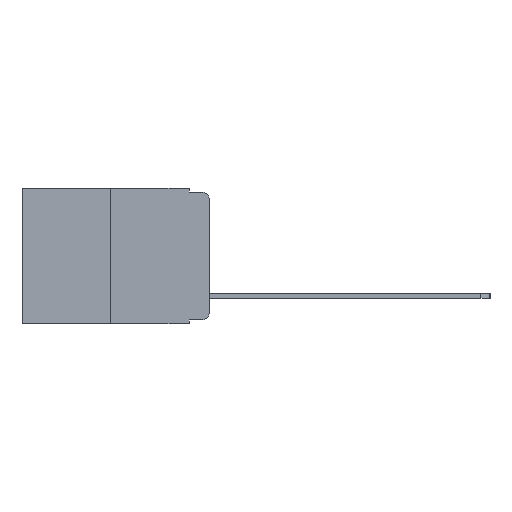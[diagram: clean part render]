
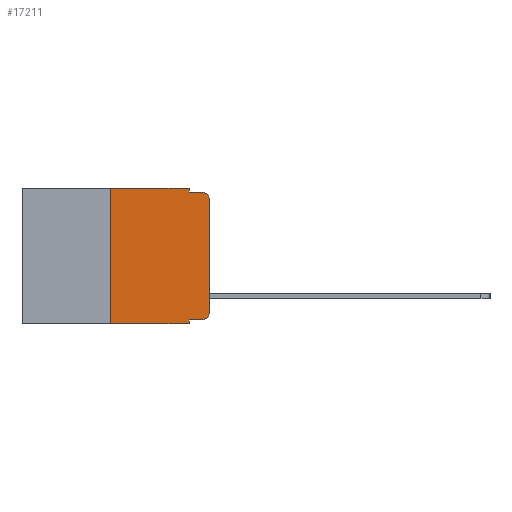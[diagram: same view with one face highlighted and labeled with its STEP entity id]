
A CAD part, left-side view. The second image highlights one B-rep face of the part: STEP entity #17211.
In plain terms, the highlighted planar face has unit normal (-1, 0, 0).
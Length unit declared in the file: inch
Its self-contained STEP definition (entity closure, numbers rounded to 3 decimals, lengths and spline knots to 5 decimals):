
#475 = CARTESIAN_POINT ( 'NONE',  ( 0., 0.051, 0. ) ) ;
#685 = EDGE_CURVE ( 'NONE', #7349, #12389, #5543, .T. ) ;
#723 = VERTEX_POINT ( 'NONE', #14719 ) ;
#1349 = LINE ( 'NONE', #15636, #16212 ) ;
#1635 = CARTESIAN_POINT ( 'NONE',  ( 0., 0.25, 0. ) ) ;
#1845 = DIRECTION ( 'NONE',  ( 1., 0., 0. ) ) ;
#1980 = DIRECTION ( 'NONE',  ( 0., 0., -1. ) ) ;
#2399 = CARTESIAN_POINT ( 'NONE',  ( 0., 0.25, -0.343 ) ) ;
#2998 = AXIS2_PLACEMENT_3D ( 'NONE', #13527, #4935, #14958 ) ;
#3083 = DIRECTION ( 'NONE',  ( -1., 0., 0. ) ) ;
#3391 = CARTESIAN_POINT ( 'NONE',  ( 0., 0.051, -0.01 ) ) ;
#3398 = DIRECTION ( 'NONE',  ( 0., 0., -1. ) ) ;
#3605 = CARTESIAN_POINT ( 'NONE',  ( 0., 0.473, 0. ) ) ;
#3629 = VERTEX_POINT ( 'NONE', #9096 ) ;
#4118 = VECTOR ( 'NONE', #17856, 39.37008 ) ;
#4158 = VECTOR ( 'NONE', #16535, 39.37008 ) ;
#4336 = ORIENTED_EDGE ( 'NONE', *, *, #8005, .T. ) ;
#4422 = ORIENTED_EDGE ( 'NONE', *, *, #9911, .T. ) ;
#4568 = LINE ( 'NONE', #3605, #4118 ) ;
#4690 = ORIENTED_EDGE ( 'NONE', *, *, #5915, .T. ) ;
#4710 = ORIENTED_EDGE ( 'NONE', *, *, #12747, .F. ) ;
#4900 = ORIENTED_EDGE ( 'NONE', *, *, #13696, .F. ) ;
#4917 = ORIENTED_EDGE ( 'NONE', *, *, #6784, .F. ) ;
#4935 = DIRECTION ( 'NONE',  ( -1., 0., 0. ) ) ;
#4967 = VERTEX_POINT ( 'NONE', #2399 ) ;
#4986 = ORIENTED_EDGE ( 'NONE', *, *, #14643, .F. ) ;
#5139 = ORIENTED_EDGE ( 'NONE', *, *, #17447, .F. ) ;
#5200 = ORIENTED_EDGE ( 'NONE', *, *, #18374, .T. ) ;
#5408 = DIRECTION ( 'NONE',  ( 0., -1., 0. ) ) ;
#5495 = ORIENTED_EDGE ( 'NONE', *, *, #685, .T. ) ;
#5543 = LINE ( 'NONE', #16844, #8527 ) ;
#5915 = EDGE_CURVE ( 'NONE', #4967, #723, #15596, .T. ) ;
#6534 = CARTESIAN_POINT ( 'NONE',  ( 0., 0.051, -0.333 ) ) ;
#6784 = EDGE_CURVE ( 'NONE', #13263, #14924, #4568, .T. ) ;
#7349 = VERTEX_POINT ( 'NONE', #7852 ) ;
#7352 = VERTEX_POINT ( 'NONE', #3391 ) ;
#7443 = CIRCLE ( 'NONE', #2998, 0.02 ) ;
#7626 = LINE ( 'NONE', #475, #18001 ) ;
#7852 = CARTESIAN_POINT ( 'NONE',  ( 0., 0., -0.313 ) ) ;
#8005 = EDGE_CURVE ( 'NONE', #3629, #7349, #7443, .T. ) ;
#8038 = LINE ( 'NONE', #10634, #15312 ) ;
#8058 = LINE ( 'NONE', #9080, #15146 ) ;
#8063 = AXIS2_PLACEMENT_3D ( 'NONE', #10509, #1845, #11990 ) ;
#8527 = VECTOR ( 'NONE', #9535, 39.37008 ) ;
#8772 = CIRCLE ( 'NONE', #9508, 0.02 ) ;
#9080 = CARTESIAN_POINT ( 'NONE',  ( 0., 0.051, -0.333 ) ) ;
#9096 = CARTESIAN_POINT ( 'NONE',  ( 0., 0.02, -0.333 ) ) ;
#9435 = VECTOR ( 'NONE', #5408, 39.37008 ) ;
#9508 = AXIS2_PLACEMENT_3D ( 'NONE', #11759, #3083, #13195 ) ;
#9535 = DIRECTION ( 'NONE',  ( 0., 0., 1. ) ) ;
#9911 = EDGE_CURVE ( 'NONE', #12325, #3629, #8058, .T. ) ;
#9995 = DIRECTION ( 'NONE',  ( 0., 0., 1. ) ) ;
#10492 = DIRECTION ( 'NONE',  ( 0., -1., 0. ) ) ;
#10509 = CARTESIAN_POINT ( 'NONE',  ( 0., 0.473, 0. ) ) ;
#10573 = PLANE ( 'NONE',  #8063 ) ;
#10634 = CARTESIAN_POINT ( 'NONE',  ( 0., 0.051, 0. ) ) ;
#11276 = EDGE_LOOP ( 'NONE', ( #5495, #5200, #5139, #4986, #4917, #4900, #4690, #4710, #4422, #4336 ) ) ;
#11724 = CARTESIAN_POINT ( 'NONE',  ( 0., 0.02, -0.01 ) ) ;
#11759 = CARTESIAN_POINT ( 'NONE',  ( 0., 0.02, -0.03 ) ) ;
#11990 = DIRECTION ( 'NONE',  ( 0., 0., -1. ) ) ;
#12325 = VERTEX_POINT ( 'NONE', #6534 ) ;
#12389 = VERTEX_POINT ( 'NONE', #13815 ) ;
#12477 = CARTESIAN_POINT ( 'NONE',  ( 0., 0.051, -0.01 ) ) ;
#12747 = EDGE_CURVE ( 'NONE', #12325, #723, #7626, .T. ) ;
#13186 = LINE ( 'NONE', #12477, #9435 ) ;
#13195 = DIRECTION ( 'NONE',  ( 0., 0., -1. ) ) ;
#13263 = VERTEX_POINT ( 'NONE', #1635 ) ;
#13527 = CARTESIAN_POINT ( 'NONE',  ( 0., 0.02, -0.313 ) ) ;
#13696 = EDGE_CURVE ( 'NONE', #4967, #13263, #1349, .T. ) ;
#13815 = CARTESIAN_POINT ( 'NONE',  ( 0., 0., -0.03 ) ) ;
#14052 = CARTESIAN_POINT ( 'NONE',  ( 0., 0.051, 0. ) ) ;
#14643 = EDGE_CURVE ( 'NONE', #14924, #7352, #8038, .T. ) ;
#14719 = CARTESIAN_POINT ( 'NONE',  ( 0., 0.051, -0.343 ) ) ;
#14924 = VERTEX_POINT ( 'NONE', #14052 ) ;
#14958 = DIRECTION ( 'NONE',  ( 0., 0., -1. ) ) ;
#15128 = CARTESIAN_POINT ( 'NONE',  ( 0., 0.473, -0.343 ) ) ;
#15146 = VECTOR ( 'NONE', #10492, 39.37008 ) ;
#15312 = VECTOR ( 'NONE', #3398, 39.37008 ) ;
#15596 = LINE ( 'NONE', #15128, #4158 ) ;
#15636 = CARTESIAN_POINT ( 'NONE',  ( 0., 0.25, 0. ) ) ;
#16212 = VECTOR ( 'NONE', #9995, 39.37008 ) ;
#16535 = DIRECTION ( 'NONE',  ( 0., -1., 0. ) ) ;
#16844 = CARTESIAN_POINT ( 'NONE',  ( 0., 0., 0. ) ) ;
#17211 = ADVANCED_FACE ( 'NONE', ( #18024 ), #10573, .F. ) ;
#17447 = EDGE_CURVE ( 'NONE', #7352, #17724, #13186, .T. ) ;
#17724 = VERTEX_POINT ( 'NONE', #11724 ) ;
#17856 = DIRECTION ( 'NONE',  ( 0., -1., 0. ) ) ;
#18001 = VECTOR ( 'NONE', #1980, 39.37008 ) ;
#18024 = FACE_OUTER_BOUND ( 'NONE', #11276, .T. ) ;
#18374 = EDGE_CURVE ( 'NONE', #12389, #17724, #8772, .T. ) ;
